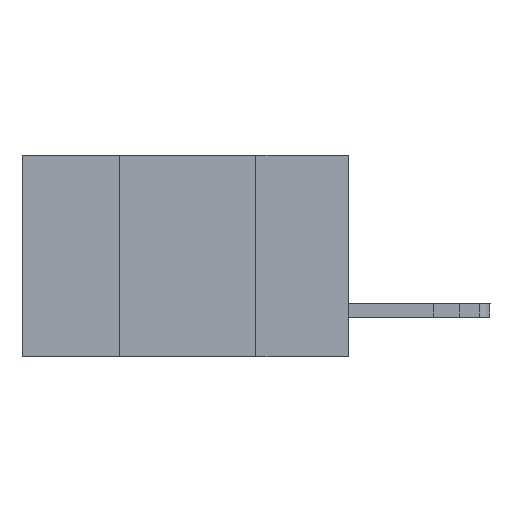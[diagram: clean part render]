
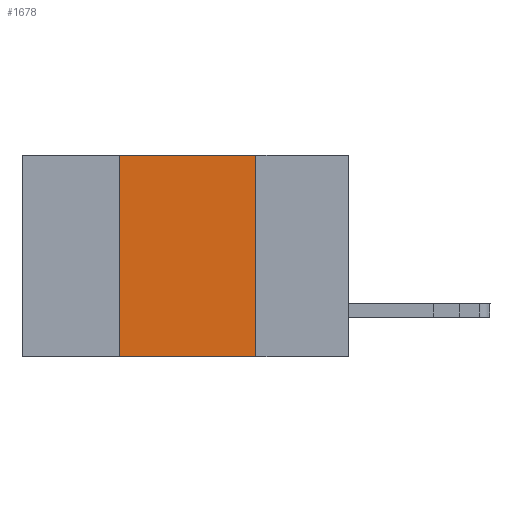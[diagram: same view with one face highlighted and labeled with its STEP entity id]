
A CAD part, left-side view. The second image highlights one B-rep face of the part: STEP entity #1678.
In plain terms, the highlighted planar face has unit normal (-1, 0, 0).
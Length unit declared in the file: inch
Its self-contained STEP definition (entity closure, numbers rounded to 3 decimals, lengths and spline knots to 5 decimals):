
#361 = EDGE_CURVE ( 'NONE', #1851, #9571, #4719, .T. ) ;
#1053 = DIRECTION ( 'NONE',  ( 0., -1., 0. ) ) ;
#1502 = DIRECTION ( 'NONE',  ( 0., -1., 0. ) ) ;
#1626 = LINE ( 'NONE', #7374, #5413 ) ;
#1678 = ADVANCED_FACE ( 'NONE', ( #9279 ), #10206, .F. ) ;
#1797 = AXIS2_PLACEMENT_3D ( 'NONE', #1979, #12383, #7108 ) ;
#1851 = VERTEX_POINT ( 'NONE', #7566 ) ;
#1979 = CARTESIAN_POINT ( 'NONE',  ( 0., 0.6, 0. ) ) ;
#3080 = VERTEX_POINT ( 'NONE', #9231 ) ;
#4102 = ORIENTED_EDGE ( 'NONE', *, *, #9303, .F. ) ;
#4106 = VERTEX_POINT ( 'NONE', #5931 ) ;
#4719 = LINE ( 'NONE', #7833, #5046 ) ;
#5046 = VECTOR ( 'NONE', #9963, 39.37008 ) ;
#5413 = VECTOR ( 'NONE', #1053, 39.37008 ) ;
#5731 = CARTESIAN_POINT ( 'NONE',  ( 0., 0.6, -0.37 ) ) ;
#5931 = CARTESIAN_POINT ( 'NONE',  ( 0., 0.17, 0. ) ) ;
#5968 = EDGE_CURVE ( 'NONE', #1851, #3080, #8177, .T. ) ;
#6671 = ORIENTED_EDGE ( 'NONE', *, *, #10373, .F. ) ;
#7108 = DIRECTION ( 'NONE',  ( 0., 0., -1. ) ) ;
#7374 = CARTESIAN_POINT ( 'NONE',  ( 0., 0.6, 0. ) ) ;
#7566 = CARTESIAN_POINT ( 'NONE',  ( 0., 0.42, -0.37 ) ) ;
#7777 = LINE ( 'NONE', #8743, #12801 ) ;
#7833 = CARTESIAN_POINT ( 'NONE',  ( 0., 0.42, 0. ) ) ;
#8177 = LINE ( 'NONE', #5731, #9452 ) ;
#8625 = EDGE_LOOP ( 'NONE', ( #6671, #4102, #12759, #9369 ) ) ;
#8743 = CARTESIAN_POINT ( 'NONE',  ( 0., 0.17, 0. ) ) ;
#9231 = CARTESIAN_POINT ( 'NONE',  ( 0., 0.17, -0.37 ) ) ;
#9279 = FACE_OUTER_BOUND ( 'NONE', #8625, .T. ) ;
#9303 = EDGE_CURVE ( 'NONE', #9571, #4106, #1626, .T. ) ;
#9369 = ORIENTED_EDGE ( 'NONE', *, *, #5968, .T. ) ;
#9452 = VECTOR ( 'NONE', #1502, 39.37008 ) ;
#9547 = DIRECTION ( 'NONE',  ( 0., 0., -1. ) ) ;
#9571 = VERTEX_POINT ( 'NONE', #9657 ) ;
#9657 = CARTESIAN_POINT ( 'NONE',  ( 0., 0.42, 0. ) ) ;
#9963 = DIRECTION ( 'NONE',  ( 0., 0., 1. ) ) ;
#10206 = PLANE ( 'NONE',  #1797 ) ;
#10373 = EDGE_CURVE ( 'NONE', #4106, #3080, #7777, .T. ) ;
#12383 = DIRECTION ( 'NONE',  ( 1., 0., 0. ) ) ;
#12759 = ORIENTED_EDGE ( 'NONE', *, *, #361, .F. ) ;
#12801 = VECTOR ( 'NONE', #9547, 39.37008 ) ;
